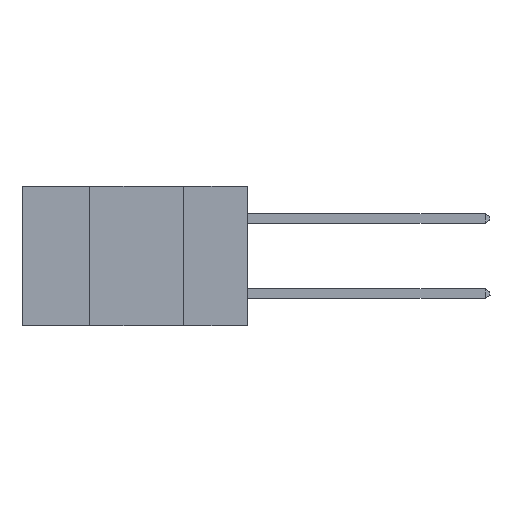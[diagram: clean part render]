
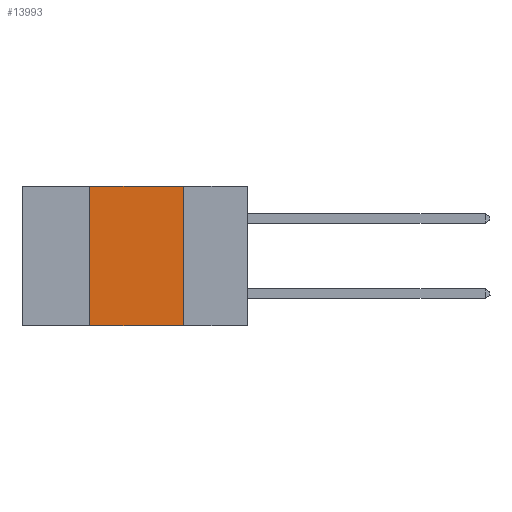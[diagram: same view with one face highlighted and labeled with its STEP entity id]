
A CAD part, left-side view. The second image highlights one B-rep face of the part: STEP entity #13993.
In plain terms, the highlighted planar face has unit normal (-1, 0, 0).
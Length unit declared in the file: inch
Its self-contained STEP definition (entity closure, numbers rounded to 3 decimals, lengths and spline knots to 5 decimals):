
#268 = VERTEX_POINT ( 'NONE', #17812 ) ;
#302 = CARTESIAN_POINT ( 'NONE',  ( 0., 0.6, -0.37 ) ) ;
#562 = LINE ( 'NONE', #22903, #20797 ) ;
#1885 = AXIS2_PLACEMENT_3D ( 'NONE', #11972, #23871, #16075 ) ;
#2573 = CARTESIAN_POINT ( 'NONE',  ( 0., 0.42, -0.37 ) ) ;
#2807 = FACE_OUTER_BOUND ( 'NONE', #4916, .T. ) ;
#4430 = DIRECTION ( 'NONE',  ( 0., 0., -1. ) ) ;
#4916 = EDGE_LOOP ( 'NONE', ( #7393, #24257, #4927, #8074 ) ) ;
#4927 = ORIENTED_EDGE ( 'NONE', *, *, #14581, .F. ) ;
#6057 = CARTESIAN_POINT ( 'NONE',  ( 0., 0.17, -0.37 ) ) ;
#6451 = EDGE_CURVE ( 'NONE', #13193, #268, #16577, .T. ) ;
#7241 = EDGE_CURVE ( 'NONE', #17224, #12829, #24465, .T. ) ;
#7393 = ORIENTED_EDGE ( 'NONE', *, *, #25710, .F. ) ;
#7579 = PLANE ( 'NONE',  #1885 ) ;
#8074 = ORIENTED_EDGE ( 'NONE', *, *, #7241, .T. ) ;
#8908 = DIRECTION ( 'NONE',  ( 0., 0., 1. ) ) ;
#11972 = CARTESIAN_POINT ( 'NONE',  ( 0., 0.6, 0. ) ) ;
#12829 = VERTEX_POINT ( 'NONE', #6057 ) ;
#13193 = VERTEX_POINT ( 'NONE', #25142 ) ;
#13993 = ADVANCED_FACE ( 'NONE', ( #2807 ), #7579, .F. ) ;
#14382 = DIRECTION ( 'NONE',  ( 0., -1., 0. ) ) ;
#14413 = DIRECTION ( 'NONE',  ( 0., -1., 0. ) ) ;
#14450 = CARTESIAN_POINT ( 'NONE',  ( 0., 0.17, 0. ) ) ;
#14581 = EDGE_CURVE ( 'NONE', #17224, #13193, #562, .T. ) ;
#15047 = LINE ( 'NONE', #14450, #17910 ) ;
#16075 = DIRECTION ( 'NONE',  ( 0., 0., -1. ) ) ;
#16577 = LINE ( 'NONE', #18450, #25772 ) ;
#17224 = VERTEX_POINT ( 'NONE', #2573 ) ;
#17812 = CARTESIAN_POINT ( 'NONE',  ( 0., 0.17, 0. ) ) ;
#17910 = VECTOR ( 'NONE', #4430, 39.37008 ) ;
#18450 = CARTESIAN_POINT ( 'NONE',  ( 0., 0.6, 0. ) ) ;
#20797 = VECTOR ( 'NONE', #8908, 39.37008 ) ;
#22903 = CARTESIAN_POINT ( 'NONE',  ( 0., 0.42, 0. ) ) ;
#23871 = DIRECTION ( 'NONE',  ( 1., 0., 0. ) ) ;
#24257 = ORIENTED_EDGE ( 'NONE', *, *, #6451, .F. ) ;
#24465 = LINE ( 'NONE', #302, #25397 ) ;
#25142 = CARTESIAN_POINT ( 'NONE',  ( 0., 0.42, 0. ) ) ;
#25397 = VECTOR ( 'NONE', #14382, 39.37008 ) ;
#25710 = EDGE_CURVE ( 'NONE', #268, #12829, #15047, .T. ) ;
#25772 = VECTOR ( 'NONE', #14413, 39.37008 ) ;
